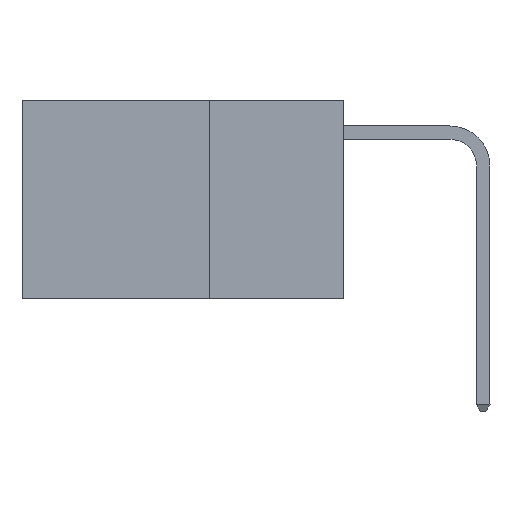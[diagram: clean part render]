
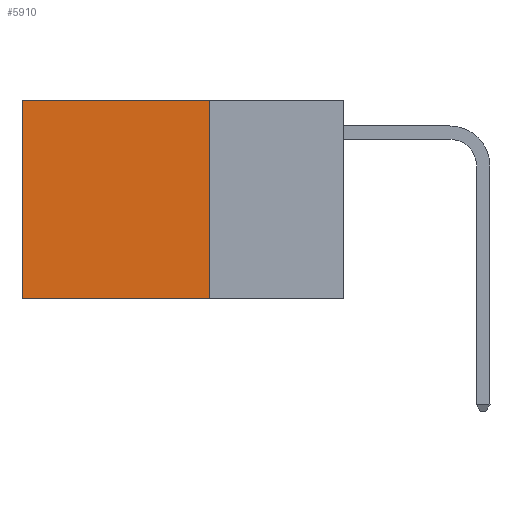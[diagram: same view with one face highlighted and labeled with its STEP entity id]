
A CAD part, left-side view. The second image highlights one B-rep face of the part: STEP entity #5910.
In plain terms, the highlighted planar face has unit normal (-1, 0, 0).
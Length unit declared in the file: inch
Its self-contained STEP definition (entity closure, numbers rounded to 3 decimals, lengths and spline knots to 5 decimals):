
#135 = EDGE_CURVE ( 'NONE', #9596, #19875, #11030, .T. ) ;
#790 = DIRECTION ( 'NONE',  ( 0., 1., 0. ) ) ;
#1016 = DIRECTION ( 'NONE',  ( 1., 0., 0. ) ) ;
#1867 = ORIENTED_EDGE ( 'NONE', *, *, #17317, .F. ) ;
#2191 = DIRECTION ( 'NONE',  ( 0., 1., 0. ) ) ;
#2375 = ORIENTED_EDGE ( 'NONE', *, *, #6296, .T. ) ;
#2700 = FACE_OUTER_BOUND ( 'NONE', #4872, .T. ) ;
#3133 = VECTOR ( 'NONE', #10845, 39.37008 ) ;
#3718 = EDGE_CURVE ( 'NONE', #18414, #21233, #17575, .T. ) ;
#4872 = EDGE_LOOP ( 'NONE', ( #2375, #9090, #1867, #19346 ) ) ;
#5878 = CARTESIAN_POINT ( 'NONE',  ( 0.2625, 0.6, 0. ) ) ;
#5910 = ADVANCED_FACE ( 'NONE', ( #2700 ), #9581, .F. ) ;
#6296 = EDGE_CURVE ( 'NONE', #21233, #19875, #21276, .T. ) ;
#7681 = VECTOR ( 'NONE', #13898, 39.37008 ) ;
#7898 = DIRECTION ( 'NONE',  ( 0., 0., -1. ) ) ;
#9090 = ORIENTED_EDGE ( 'NONE', *, *, #135, .F. ) ;
#9171 = CARTESIAN_POINT ( 'NONE',  ( 0.2625, 0.6, 0. ) ) ;
#9364 = CARTESIAN_POINT ( 'NONE',  ( 0.2625, 0.25, -0.37 ) ) ;
#9581 = PLANE ( 'NONE',  #16756 ) ;
#9596 = VERTEX_POINT ( 'NONE', #13186 ) ;
#10845 = DIRECTION ( 'NONE',  ( 0., 0., -1. ) ) ;
#11030 = LINE ( 'NONE', #9364, #16453 ) ;
#12565 = CARTESIAN_POINT ( 'NONE',  ( 0.2625, 0.25, 0. ) ) ;
#13186 = CARTESIAN_POINT ( 'NONE',  ( 0.2625, 0.25, -0.37 ) ) ;
#13500 = VECTOR ( 'NONE', #2191, 39.37008 ) ;
#13898 = DIRECTION ( 'NONE',  ( 0., 0., -1. ) ) ;
#14095 = CARTESIAN_POINT ( 'NONE',  ( 0.2625, 0.25, 0. ) ) ;
#14218 = CARTESIAN_POINT ( 'NONE',  ( 0.2625, 0.25, 0. ) ) ;
#16396 = CARTESIAN_POINT ( 'NONE',  ( 0.2625, 0.25, 0. ) ) ;
#16453 = VECTOR ( 'NONE', #790, 39.37008 ) ;
#16756 = AXIS2_PLACEMENT_3D ( 'NONE', #16396, #1016, #7898 ) ;
#17272 = LINE ( 'NONE', #14218, #7681 ) ;
#17317 = EDGE_CURVE ( 'NONE', #18414, #9596, #17272, .T. ) ;
#17575 = LINE ( 'NONE', #14095, #13500 ) ;
#18414 = VERTEX_POINT ( 'NONE', #12565 ) ;
#19346 = ORIENTED_EDGE ( 'NONE', *, *, #3718, .T. ) ;
#19764 = CARTESIAN_POINT ( 'NONE',  ( 0.2625, 0.6, -0.37 ) ) ;
#19875 = VERTEX_POINT ( 'NONE', #19764 ) ;
#21233 = VERTEX_POINT ( 'NONE', #5878 ) ;
#21276 = LINE ( 'NONE', #9171, #3133 ) ;
